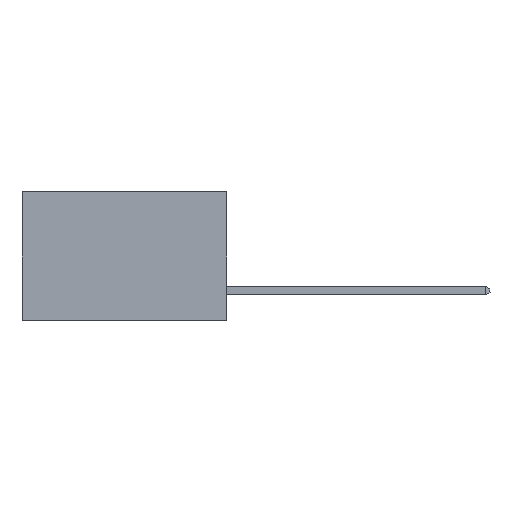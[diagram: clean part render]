
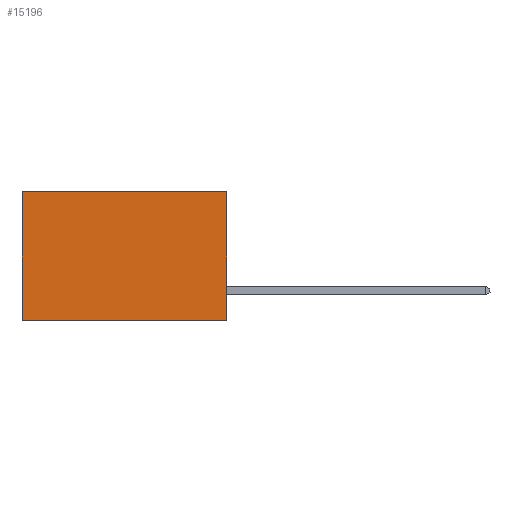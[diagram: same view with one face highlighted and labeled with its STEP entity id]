
A CAD part, left-side view. The second image highlights one B-rep face of the part: STEP entity #15196.
In plain terms, the highlighted planar face has unit normal (-1, 0, 0).
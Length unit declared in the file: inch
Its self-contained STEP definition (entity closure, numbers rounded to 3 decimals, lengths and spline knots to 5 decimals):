
#131 = ORIENTED_EDGE ( 'NONE', *, *, #6046, .F. ) ;
#2627 = AXIS2_PLACEMENT_3D ( 'NONE', #13583, #6143, #14807 ) ;
#2915 = VECTOR ( 'NONE', #8679, 39.37008 ) ;
#2970 = VECTOR ( 'NONE', #14251, 39.37008 ) ;
#3539 = ORIENTED_EDGE ( 'NONE', *, *, #8659, .T. ) ;
#4420 = CARTESIAN_POINT ( 'NONE',  ( 0.277, 0.59, -0.37 ) ) ;
#4727 = DIRECTION ( 'NONE',  ( 0., 0., -1. ) ) ;
#4934 = EDGE_LOOP ( 'NONE', ( #3539, #131, #6621, #8958 ) ) ;
#5553 = CARTESIAN_POINT ( 'NONE',  ( 0.277, 0.59, 0. ) ) ;
#5848 = VERTEX_POINT ( 'NONE', #10231 ) ;
#6046 = EDGE_CURVE ( 'NONE', #15503, #6123, #9564, .T. ) ;
#6123 = VERTEX_POINT ( 'NONE', #8016 ) ;
#6143 = DIRECTION ( 'NONE',  ( 1., 0., 0. ) ) ;
#6171 = LINE ( 'NONE', #4420, #9098 ) ;
#6235 = FACE_OUTER_BOUND ( 'NONE', #4934, .T. ) ;
#6302 = LINE ( 'NONE', #14432, #2970 ) ;
#6621 = ORIENTED_EDGE ( 'NONE', *, *, #10541, .F. ) ;
#7369 = PLANE ( 'NONE',  #2627 ) ;
#8016 = CARTESIAN_POINT ( 'NONE',  ( 0.277, 0.59, -0.37 ) ) ;
#8602 = CARTESIAN_POINT ( 'NONE',  ( 0.277, 0., -0.37 ) ) ;
#8659 = EDGE_CURVE ( 'NONE', #10158, #6123, #6171, .T. ) ;
#8679 = DIRECTION ( 'NONE',  ( 0., 1., 0. ) ) ;
#8958 = ORIENTED_EDGE ( 'NONE', *, *, #14136, .T. ) ;
#9098 = VECTOR ( 'NONE', #4727, 39.37008 ) ;
#9564 = LINE ( 'NONE', #8602, #2915 ) ;
#9795 = LINE ( 'NONE', #12953, #15950 ) ;
#10158 = VERTEX_POINT ( 'NONE', #5553 ) ;
#10231 = CARTESIAN_POINT ( 'NONE',  ( 0.277, 0., 0. ) ) ;
#10541 = EDGE_CURVE ( 'NONE', #5848, #15503, #6302, .T. ) ;
#11733 = CARTESIAN_POINT ( 'NONE',  ( 0.277, 0., -0.37 ) ) ;
#12953 = CARTESIAN_POINT ( 'NONE',  ( 0.277, 0., 0. ) ) ;
#13583 = CARTESIAN_POINT ( 'NONE',  ( 0.277, 0., -0.37 ) ) ;
#14136 = EDGE_CURVE ( 'NONE', #5848, #10158, #9795, .T. ) ;
#14171 = DIRECTION ( 'NONE',  ( 0., 1., 0. ) ) ;
#14251 = DIRECTION ( 'NONE',  ( 0., 0., -1. ) ) ;
#14432 = CARTESIAN_POINT ( 'NONE',  ( 0.277, 0., -0.37 ) ) ;
#14807 = DIRECTION ( 'NONE',  ( 0., 0., -1. ) ) ;
#15196 = ADVANCED_FACE ( 'NONE', ( #6235 ), #7369, .F. ) ;
#15503 = VERTEX_POINT ( 'NONE', #11733 ) ;
#15950 = VECTOR ( 'NONE', #14171, 39.37008 ) ;
